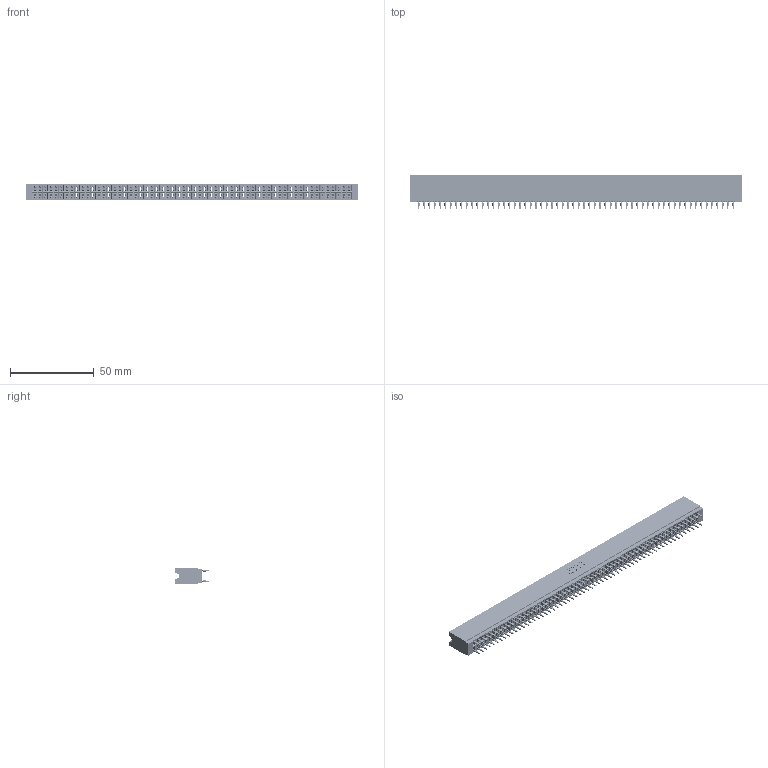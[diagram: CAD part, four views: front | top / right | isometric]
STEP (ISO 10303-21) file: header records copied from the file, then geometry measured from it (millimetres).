
FILE_DESCRIPTION (( 'STEP AP203' ), '1' );
FILE_NAME ('746-120-560-206.STEP', '2026-03-06T17:53:26', ( '' ), ( '' ), 'SwSTEP 2.0', 'SolidWorks 2023', '' );
FILE_SCHEMA (( 'CONFIG_CONTROL_DESIGN' ));
Length unit declared in the file: millimetre
Products named in the file (3): 746 Part_.515 Slot Depth - 06; 746-120-560-206; 746-292-001_560
Assembly tree (121 placements, depth 2):
  746-120-560-206
    746 Part_.515 Slot Depth - 06
    746-292-001_560  x120
Bounding box: 197.74 x 20.82 x 9.91 mm (x, y, z)
Volume: 21472.4 mm3; surface area: 36815.1 mm2
Topology: 121 solids, 121 shells, 11438 faces, 31825 edges, 20395 vertices
Faces by surface type: plane 5696, cylinder 2622, bspline 2400, torus 720
Entity records: 90256 total; most frequent: CARTESIAN_POINT 17782, ORIENTED_EDGE 15574, DIRECTION 12979, EDGE_CURVE 7787, VECTOR 6995, LINE 6995, VERTEX_POINT 5163, AXIS2_PLACEMENT_3D 2992
